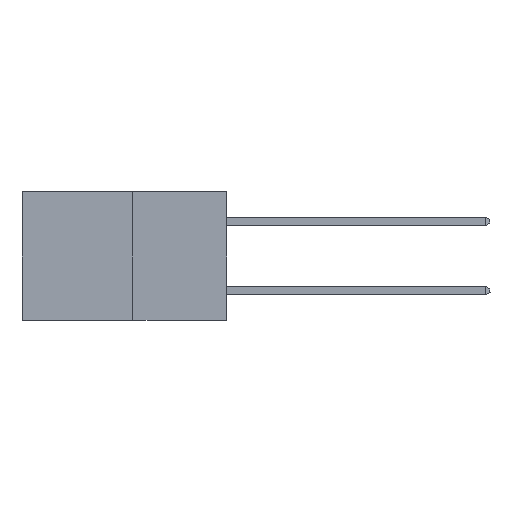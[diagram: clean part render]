
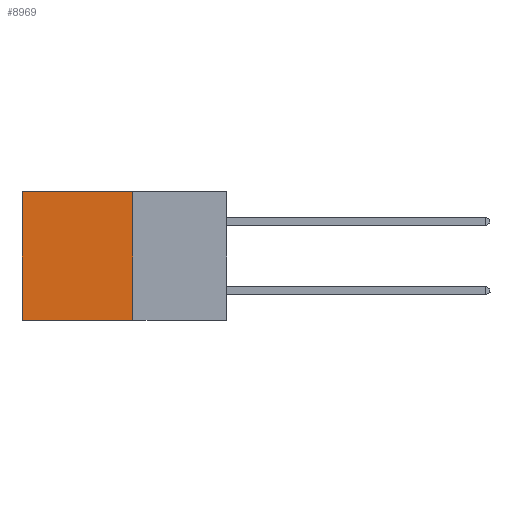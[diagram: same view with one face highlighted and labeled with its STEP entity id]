
A CAD part, left-side view. The second image highlights one B-rep face of the part: STEP entity #8969.
In plain terms, the highlighted planar face has unit normal (-1, 0, 0).
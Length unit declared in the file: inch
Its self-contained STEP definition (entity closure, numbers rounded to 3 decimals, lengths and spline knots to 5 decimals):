
#479 = CARTESIAN_POINT ( 'NONE',  ( 0.277, 0.27, 0. ) ) ;
#1373 = VERTEX_POINT ( 'NONE', #11267 ) ;
#1401 = EDGE_LOOP ( 'NONE', ( #21263, #10554, #5540, #23367 ) ) ;
#1699 = CARTESIAN_POINT ( 'NONE',  ( 0.277, 0.27, -0.37 ) ) ;
#2851 = LINE ( 'NONE', #14025, #23902 ) ;
#3408 = CARTESIAN_POINT ( 'NONE',  ( 0.277, 0.27, -0.37 ) ) ;
#3671 = EDGE_CURVE ( 'NONE', #1373, #16145, #2851, .T. ) ;
#3898 = CARTESIAN_POINT ( 'NONE',  ( 0.277, 0.27, 0. ) ) ;
#3919 = AXIS2_PLACEMENT_3D ( 'NONE', #15544, #8512, #8463 ) ;
#4717 = EDGE_CURVE ( 'NONE', #18653, #16145, #10877, .T. ) ;
#5540 = ORIENTED_EDGE ( 'NONE', *, *, #10575, .F. ) ;
#6039 = VECTOR ( 'NONE', #16012, 39.37008 ) ;
#8463 = DIRECTION ( 'NONE',  ( 0., 0., -1. ) ) ;
#8512 = DIRECTION ( 'NONE',  ( 1., 0., 0. ) ) ;
#8969 = ADVANCED_FACE ( 'NONE', ( #11323 ), #15618, .F. ) ;
#10554 = ORIENTED_EDGE ( 'NONE', *, *, #4717, .F. ) ;
#10575 = EDGE_CURVE ( 'NONE', #15505, #18653, #10647, .T. ) ;
#10647 = LINE ( 'NONE', #17896, #15924 ) ;
#10863 = LINE ( 'NONE', #3898, #6039 ) ;
#10877 = LINE ( 'NONE', #1699, #15520 ) ;
#11267 = CARTESIAN_POINT ( 'NONE',  ( 0.277, 0.59, 0. ) ) ;
#11323 = FACE_OUTER_BOUND ( 'NONE', #1401, .T. ) ;
#14025 = CARTESIAN_POINT ( 'NONE',  ( 0.277, 0.59, -0.37 ) ) ;
#15505 = VERTEX_POINT ( 'NONE', #479 ) ;
#15520 = VECTOR ( 'NONE', #25590, 39.37008 ) ;
#15544 = CARTESIAN_POINT ( 'NONE',  ( 0.277, 0.27, -0.37 ) ) ;
#15618 = PLANE ( 'NONE',  #3919 ) ;
#15924 = VECTOR ( 'NONE', #17891, 39.37008 ) ;
#16012 = DIRECTION ( 'NONE',  ( 0., 1., 0. ) ) ;
#16145 = VERTEX_POINT ( 'NONE', #22580 ) ;
#17891 = DIRECTION ( 'NONE',  ( 0., 0., -1. ) ) ;
#17896 = CARTESIAN_POINT ( 'NONE',  ( 0.277, 0.27, -0.37 ) ) ;
#18653 = VERTEX_POINT ( 'NONE', #3408 ) ;
#18881 = DIRECTION ( 'NONE',  ( 0., 0., -1. ) ) ;
#21263 = ORIENTED_EDGE ( 'NONE', *, *, #3671, .T. ) ;
#22580 = CARTESIAN_POINT ( 'NONE',  ( 0.277, 0.59, -0.37 ) ) ;
#23312 = EDGE_CURVE ( 'NONE', #15505, #1373, #10863, .T. ) ;
#23367 = ORIENTED_EDGE ( 'NONE', *, *, #23312, .T. ) ;
#23902 = VECTOR ( 'NONE', #18881, 39.37008 ) ;
#25590 = DIRECTION ( 'NONE',  ( 0., 1., 0. ) ) ;
